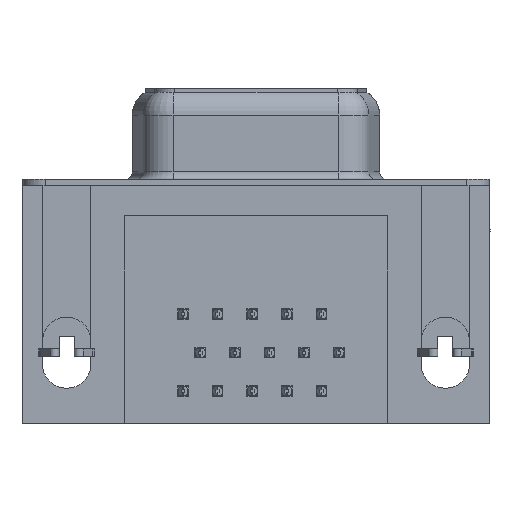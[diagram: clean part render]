
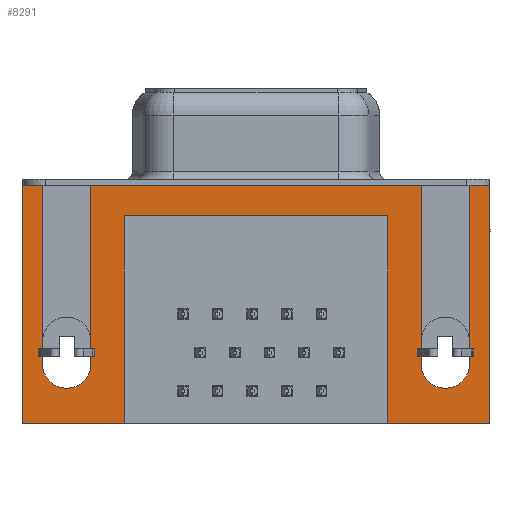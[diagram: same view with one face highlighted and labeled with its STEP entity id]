
A CAD part, front view. The second image highlights one B-rep face of the part: STEP entity #8291.
In plain terms, the highlighted planar face has unit normal (0, -1, 0).
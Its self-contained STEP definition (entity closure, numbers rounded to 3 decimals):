
#165 = LINE ( 'NONE', #32051, #37311 ) ;
#197 = VERTEX_POINT ( 'NONE', #19910 ) ;
#214 = CARTESIAN_POINT ( 'NONE',  ( 27.9, -6.275, -15.7 ) ) ;
#1401 = DIRECTION ( 'NONE',  ( 0., -1., 0. ) ) ;
#1441 = CARTESIAN_POINT ( 'NONE',  ( -2.91, -6.275, -2.5 ) ) ;
#2054 = DIRECTION ( 'NONE',  ( 0., 0., -1. ) ) ;
#2337 = EDGE_LOOP ( 'NONE', ( #5516, #5919, #29302, #33431, #18321, #12835, #12126, #14683, #16709, #7294, #15867, #34538, #19773, #23177, #36635, #24658 ) ) ;
#3364 = LINE ( 'NONE', #15028, #11101 ) ;
#3650 = VERTEX_POINT ( 'NONE', #14635 ) ;
#4776 = DIRECTION ( 'NONE',  ( 0., -1., 0. ) ) ;
#5516 = ORIENTED_EDGE ( 'NONE', *, *, #15666, .F. ) ;
#5766 = CARTESIAN_POINT ( 'NONE',  ( 21.2, -6.275, -2. ) ) ;
#5877 = CARTESIAN_POINT ( 'NONE',  ( -2.91, -6.275, 0. ) ) ;
#5919 = ORIENTED_EDGE ( 'NONE', *, *, #15720, .F. ) ;
#5983 = VERTEX_POINT ( 'NONE', #29618 ) ;
#6591 = DIRECTION ( 'NONE',  ( 0., 0., -1. ) ) ;
#6710 = CARTESIAN_POINT ( 'NONE',  ( -2.91, -6.275, -2.5 ) ) ;
#7294 = ORIENTED_EDGE ( 'NONE', *, *, #16165, .F. ) ;
#7515 = VECTOR ( 'NONE', #27301, 1000. ) ;
#7527 = EDGE_CURVE ( 'NONE', #9079, #23203, #15813, .T. ) ;
#7784 = CARTESIAN_POINT ( 'NONE',  ( 27.9, -6.275, -2.5 ) ) ;
#7878 = VERTEX_POINT ( 'NONE', #15087 ) ;
#7944 = LINE ( 'NONE', #19415, #23391 ) ;
#8291 = ADVANCED_FACE ( 'NONE', ( #35660 ), #10236, .T. ) ;
#8422 = EDGE_CURVE ( 'NONE', #21561, #23249, #31952, .T. ) ;
#8796 = DIRECTION ( 'NONE',  ( 1., 0., 0. ) ) ;
#8953 = LINE ( 'NONE', #6710, #22565 ) ;
#9063 = EDGE_CURVE ( 'NONE', #32779, #11040, #31004, .T. ) ;
#9079 = VERTEX_POINT ( 'NONE', #20548 ) ;
#9291 = LINE ( 'NONE', #21006, #10202 ) ;
#9308 = CARTESIAN_POINT ( 'NONE',  ( -1.6, -6.275, 0. ) ) ;
#9601 = EDGE_CURVE ( 'NONE', #23469, #197, #17083, .T. ) ;
#9742 = VERTEX_POINT ( 'NONE', #15525 ) ;
#10202 = VECTOR ( 'NONE', #6591, 1000. ) ;
#10236 = PLANE ( 'NONE',  #10591 ) ;
#10255 = CARTESIAN_POINT ( 'NONE',  ( 26.59, -6.275, 0. ) ) ;
#10591 = AXIS2_PLACEMENT_3D ( 'NONE', #1441, #30782, #13180 ) ;
#11040 = VERTEX_POINT ( 'NONE', #9308 ) ;
#11101 = VECTOR ( 'NONE', #35667, 1000. ) ;
#12126 = ORIENTED_EDGE ( 'NONE', *, *, #16105, .F. ) ;
#12642 = CARTESIAN_POINT ( 'NONE',  ( 27.9, -6.275, -15.7 ) ) ;
#12835 = ORIENTED_EDGE ( 'NONE', *, *, #7527, .F. ) ;
#13180 = DIRECTION ( 'NONE',  ( 0., 0., -1. ) ) ;
#14008 = CARTESIAN_POINT ( 'NONE',  ( 3.79, -6.275, -2. ) ) ;
#14635 = CARTESIAN_POINT ( 'NONE',  ( 3.79, -6.275, -2. ) ) ;
#14683 = ORIENTED_EDGE ( 'NONE', *, *, #9063, .F. ) ;
#14708 = EDGE_CURVE ( 'NONE', #9742, #32779, #8953, .T. ) ;
#14711 = LINE ( 'NONE', #14008, #37272 ) ;
#15028 = CARTESIAN_POINT ( 'NONE',  ( 1.6, -6.275, 0. ) ) ;
#15043 = CARTESIAN_POINT ( 'NONE',  ( -2.91, -6.275, 0. ) ) ;
#15087 = CARTESIAN_POINT ( 'NONE',  ( 21.2, -6.275, -15.7 ) ) ;
#15168 = LINE ( 'NONE', #12642, #7515 ) ;
#15185 = EDGE_CURVE ( 'NONE', #30960, #23249, #34168, .T. ) ;
#15198 = VECTOR ( 'NONE', #30803, 1000. ) ;
#15525 = CARTESIAN_POINT ( 'NONE',  ( -2.91, -6.275, -15.7 ) ) ;
#15666 = EDGE_CURVE ( 'NONE', #16992, #21561, #37768, .T. ) ;
#15720 = EDGE_CURVE ( 'NONE', #24471, #16992, #35970, .T. ) ;
#15813 = CIRCLE ( 'NONE', #18855, 1.6 ) ;
#15867 = ORIENTED_EDGE ( 'NONE', *, *, #16379, .F. ) ;
#15935 = EDGE_CURVE ( 'NONE', #197, #24471, #165, .T. ) ;
#16053 = EDGE_CURVE ( 'NONE', #23203, #23469, #3364, .T. ) ;
#16105 = EDGE_CURVE ( 'NONE', #11040, #9079, #9291, .T. ) ;
#16146 = VECTOR ( 'NONE', #32703, 1000. ) ;
#16165 = EDGE_CURVE ( 'NONE', #23524, #9742, #15168, .T. ) ;
#16379 = EDGE_CURVE ( 'NONE', #3650, #23524, #7944, .T. ) ;
#16438 = EDGE_CURVE ( 'NONE', #5983, #3650, #14711, .T. ) ;
#16560 = EDGE_CURVE ( 'NONE', #7878, #5983, #35467, .T. ) ;
#16621 = EDGE_CURVE ( 'NONE', #30960, #7878, #23844, .T. ) ;
#16709 = ORIENTED_EDGE ( 'NONE', *, *, #14708, .F. ) ;
#16778 = DIRECTION ( 'NONE',  ( 1., 0., 0. ) ) ;
#16992 = VERTEX_POINT ( 'NONE', #27215 ) ;
#17083 = LINE ( 'NONE', #15043, #16146 ) ;
#17193 = CARTESIAN_POINT ( 'NONE',  ( 27.9, -6.275, -15.7 ) ) ;
#17865 = CARTESIAN_POINT ( 'NONE',  ( 27.9, -6.275, 0. ) ) ;
#18321 = ORIENTED_EDGE ( 'NONE', *, *, #16053, .F. ) ;
#18406 = VECTOR ( 'NONE', #28277, 1000. ) ;
#18801 = CARTESIAN_POINT ( 'NONE',  ( 0., -6.275, -11.78 ) ) ;
#18855 = AXIS2_PLACEMENT_3D ( 'NONE', #18801, #1401, #21774 ) ;
#19415 = CARTESIAN_POINT ( 'NONE',  ( 3.79, -6.275, -2. ) ) ;
#19723 = AXIS2_PLACEMENT_3D ( 'NONE', #22213, #4776, #25223 ) ;
#19773 = ORIENTED_EDGE ( 'NONE', *, *, #16560, .F. ) ;
#19910 = CARTESIAN_POINT ( 'NONE',  ( 23.39, -6.275, 0. ) ) ;
#20548 = CARTESIAN_POINT ( 'NONE',  ( -1.6, -6.275, -11.78 ) ) ;
#20571 = DIRECTION ( 'NONE',  ( -1., 0., 0. ) ) ;
#21006 = CARTESIAN_POINT ( 'NONE',  ( -1.6, -6.275, 0. ) ) ;
#21561 = VERTEX_POINT ( 'NONE', #25516 ) ;
#21774 = DIRECTION ( 'NONE',  ( 1., 0., 0. ) ) ;
#22213 = CARTESIAN_POINT ( 'NONE',  ( 24.99, -6.275, -11.78 ) ) ;
#22565 = VECTOR ( 'NONE', #24252, 1000. ) ;
#23177 = ORIENTED_EDGE ( 'NONE', *, *, #16621, .F. ) ;
#23203 = VERTEX_POINT ( 'NONE', #35484 ) ;
#23249 = VERTEX_POINT ( 'NONE', #17865 ) ;
#23391 = VECTOR ( 'NONE', #2054, 1000. ) ;
#23469 = VERTEX_POINT ( 'NONE', #25237 ) ;
#23524 = VERTEX_POINT ( 'NONE', #37225 ) ;
#23844 = LINE ( 'NONE', #214, #33608 ) ;
#24252 = DIRECTION ( 'NONE',  ( 0., 0., 1. ) ) ;
#24471 = VERTEX_POINT ( 'NONE', #28144 ) ;
#24658 = ORIENTED_EDGE ( 'NONE', *, *, #8422, .F. ) ;
#25223 = DIRECTION ( 'NONE',  ( -1., 0., 0. ) ) ;
#25237 = CARTESIAN_POINT ( 'NONE',  ( 1.6, -6.275, 0. ) ) ;
#25463 = CARTESIAN_POINT ( 'NONE',  ( -2.91, -6.275, 0. ) ) ;
#25516 = CARTESIAN_POINT ( 'NONE',  ( 26.59, -6.275, 0. ) ) ;
#26214 = DIRECTION ( 'NONE',  ( 0., 0., 1. ) ) ;
#26747 = CARTESIAN_POINT ( 'NONE',  ( -2.91, -6.275, 0. ) ) ;
#27215 = CARTESIAN_POINT ( 'NONE',  ( 26.59, -6.275, -11.78 ) ) ;
#27301 = DIRECTION ( 'NONE',  ( -1., 0., 0. ) ) ;
#28144 = CARTESIAN_POINT ( 'NONE',  ( 23.39, -6.275, -11.78 ) ) ;
#28277 = DIRECTION ( 'NONE',  ( 0., 0., 1. ) ) ;
#29302 = ORIENTED_EDGE ( 'NONE', *, *, #15935, .F. ) ;
#29618 = CARTESIAN_POINT ( 'NONE',  ( 21.2, -6.275, -2. ) ) ;
#30782 = DIRECTION ( 'NONE',  ( 0., -1., 0. ) ) ;
#30803 = DIRECTION ( 'NONE',  ( 0., 0., 1. ) ) ;
#30960 = VERTEX_POINT ( 'NONE', #17193 ) ;
#31004 = LINE ( 'NONE', #5877, #37853 ) ;
#31046 = VECTOR ( 'NONE', #16778, 1000. ) ;
#31621 = DIRECTION ( 'NONE',  ( -1., 0., 0. ) ) ;
#31952 = LINE ( 'NONE', #25463, #31046 ) ;
#32051 = CARTESIAN_POINT ( 'NONE',  ( 23.39, -6.275, 0. ) ) ;
#32703 = DIRECTION ( 'NONE',  ( 1., 0., 0. ) ) ;
#32779 = VERTEX_POINT ( 'NONE', #26747 ) ;
#33431 = ORIENTED_EDGE ( 'NONE', *, *, #9601, .F. ) ;
#33608 = VECTOR ( 'NONE', #20571, 1000. ) ;
#34168 = LINE ( 'NONE', #7784, #18406 ) ;
#34516 = VECTOR ( 'NONE', #26214, 1000. ) ;
#34538 = ORIENTED_EDGE ( 'NONE', *, *, #16438, .F. ) ;
#34904 = DIRECTION ( 'NONE',  ( 0., 0., -1. ) ) ;
#35467 = LINE ( 'NONE', #5766, #34516 ) ;
#35484 = CARTESIAN_POINT ( 'NONE',  ( 1.6, -6.275, -11.78 ) ) ;
#35660 = FACE_OUTER_BOUND ( 'NONE', #2337, .T. ) ;
#35667 = DIRECTION ( 'NONE',  ( 0., 0., 1. ) ) ;
#35970 = CIRCLE ( 'NONE', #19723, 1.6 ) ;
#36635 = ORIENTED_EDGE ( 'NONE', *, *, #15185, .T. ) ;
#37225 = CARTESIAN_POINT ( 'NONE',  ( 3.79, -6.275, -15.7 ) ) ;
#37272 = VECTOR ( 'NONE', #31621, 1000. ) ;
#37311 = VECTOR ( 'NONE', #34904, 1000. ) ;
#37768 = LINE ( 'NONE', #10255, #15198 ) ;
#37853 = VECTOR ( 'NONE', #8796, 1000. ) ;
